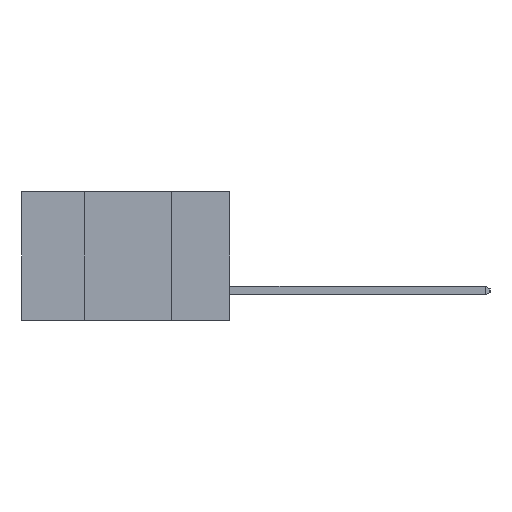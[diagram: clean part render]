
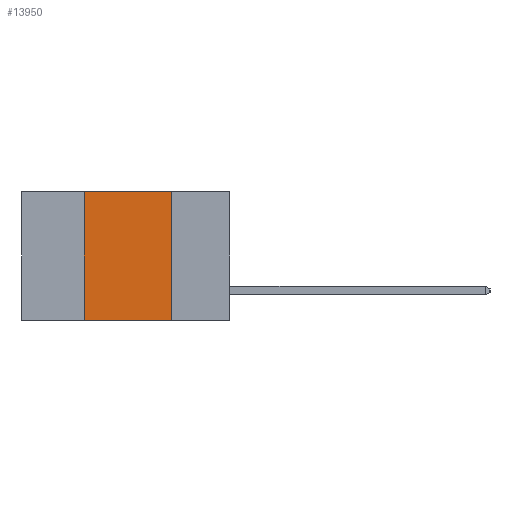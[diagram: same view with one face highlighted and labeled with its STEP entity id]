
A CAD part, left-side view. The second image highlights one B-rep face of the part: STEP entity #13950.
In plain terms, the highlighted planar face has unit normal (-1, 0, 0).
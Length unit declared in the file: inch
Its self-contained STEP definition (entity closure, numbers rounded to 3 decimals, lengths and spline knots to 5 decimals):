
#975 = VERTEX_POINT ( 'NONE', #10489 ) ;
#2326 = EDGE_CURVE ( 'NONE', #9749, #8234, #5966, .T. ) ;
#2572 = VECTOR ( 'NONE', #7152, 39.37008 ) ;
#2970 = ORIENTED_EDGE ( 'NONE', *, *, #15492, .F. ) ;
#3187 = EDGE_CURVE ( 'NONE', #9749, #975, #8453, .T. ) ;
#3297 = VECTOR ( 'NONE', #3567, 39.37008 ) ;
#3406 = CARTESIAN_POINT ( 'NONE',  ( 0., 0.6, -0.37 ) ) ;
#3567 = DIRECTION ( 'NONE',  ( 0., -1., 0. ) ) ;
#4096 = AXIS2_PLACEMENT_3D ( 'NONE', #15867, #6053, #14742 ) ;
#4325 = DIRECTION ( 'NONE',  ( 0., 0., -1. ) ) ;
#5077 = CARTESIAN_POINT ( 'NONE',  ( 0., 0.42, -0.37 ) ) ;
#5966 = LINE ( 'NONE', #3406, #2572 ) ;
#6053 = DIRECTION ( 'NONE',  ( 1., 0., 0. ) ) ;
#6312 = DIRECTION ( 'NONE',  ( 0., 0., 1. ) ) ;
#6641 = LINE ( 'NONE', #12266, #3297 ) ;
#7152 = DIRECTION ( 'NONE',  ( 0., -1., 0. ) ) ;
#7659 = CARTESIAN_POINT ( 'NONE',  ( 0., 0.17, -0.37 ) ) ;
#8166 = LINE ( 'NONE', #14293, #11519 ) ;
#8234 = VERTEX_POINT ( 'NONE', #7659 ) ;
#8237 = CARTESIAN_POINT ( 'NONE',  ( 0., 0.17, 0. ) ) ;
#8453 = LINE ( 'NONE', #5077, #14397 ) ;
#9264 = EDGE_LOOP ( 'NONE', ( #9824, #2970, #14135, #14447 ) ) ;
#9749 = VERTEX_POINT ( 'NONE', #13264 ) ;
#9824 = ORIENTED_EDGE ( 'NONE', *, *, #14540, .F. ) ;
#10489 = CARTESIAN_POINT ( 'NONE',  ( 0., 0.42, 0. ) ) ;
#11519 = VECTOR ( 'NONE', #4325, 39.37008 ) ;
#12266 = CARTESIAN_POINT ( 'NONE',  ( 0., 0.6, 0. ) ) ;
#13264 = CARTESIAN_POINT ( 'NONE',  ( 0., 0.42, -0.37 ) ) ;
#13495 = PLANE ( 'NONE',  #4096 ) ;
#13950 = ADVANCED_FACE ( 'NONE', ( #14315 ), #13495, .F. ) ;
#14135 = ORIENTED_EDGE ( 'NONE', *, *, #3187, .F. ) ;
#14293 = CARTESIAN_POINT ( 'NONE',  ( 0., 0.17, -0.37 ) ) ;
#14315 = FACE_OUTER_BOUND ( 'NONE', #9264, .T. ) ;
#14397 = VECTOR ( 'NONE', #6312, 39.37008 ) ;
#14447 = ORIENTED_EDGE ( 'NONE', *, *, #2326, .T. ) ;
#14540 = EDGE_CURVE ( 'NONE', #15383, #8234, #8166, .T. ) ;
#14742 = DIRECTION ( 'NONE',  ( 0., 0., -1. ) ) ;
#15383 = VERTEX_POINT ( 'NONE', #8237 ) ;
#15492 = EDGE_CURVE ( 'NONE', #975, #15383, #6641, .T. ) ;
#15867 = CARTESIAN_POINT ( 'NONE',  ( 0., 0.6, 0. ) ) ;
